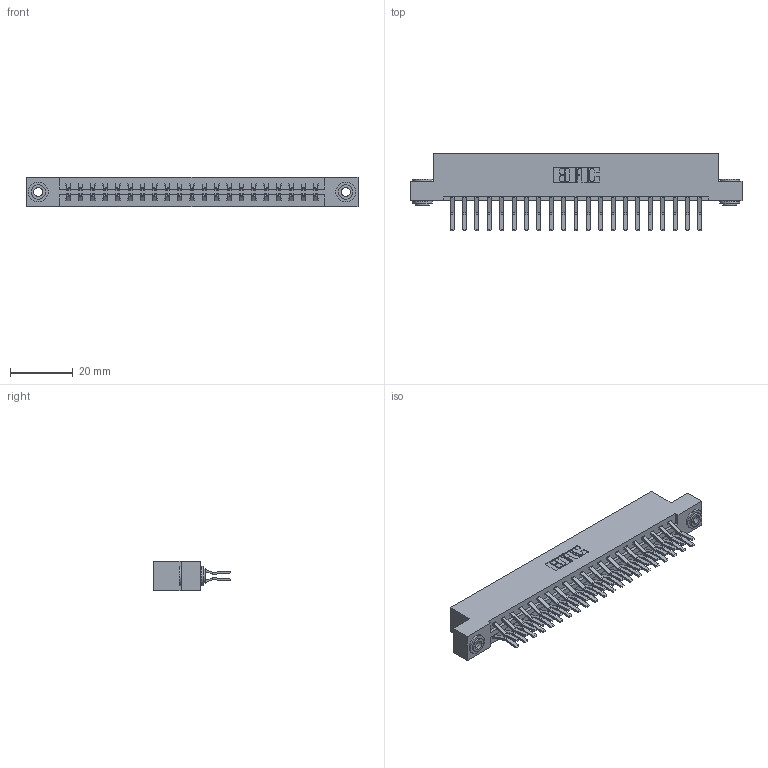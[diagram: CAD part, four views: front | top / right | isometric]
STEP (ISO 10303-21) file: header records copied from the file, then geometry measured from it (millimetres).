
FILE_DESCRIPTION (( 'STEP AP203' ), '1' );
FILE_NAME ('387-042-560-203.STEP', '2019-10-18T04:57:47', ( '' ), ( '' ), 'SwSTEP 2.0', 'SolidWorks 2016', '' );
FILE_SCHEMA (( 'CONFIG_CONTROL_DESIGN' ));
Length unit declared in the file: inch
Products named in the file (4): 337 Part_Flush Mounting Lugs - 0.156 Dia-TH; 387-042-560-203; 345-292-001_560 Tail; 345-250-002_345-250-002-102
Assembly tree (45 placements, depth 2):
  387-042-560-203
    337 Part_Flush Mounting Lugs - 0.156 Dia-TH
    345-292-001_560 Tail  x42
    345-250-002_345-250-002-102  x2
Bounding box: 106.22 x 24.78 x 9.4 mm (x, y, z)
Volume: 11209.8 mm3; surface area: 13489.8 mm2
Topology: 45 solids, 45 shells, 2504 faces, 7401 edges, 4874 vertices
Faces by surface type: plane 1676, cylinder 820, cone 8
Entity records: 19736 total; most frequent: CARTESIAN_POINT 3317, ORIENTED_EDGE 3246, DIRECTION 2897, EDGE_CURVE 1623, LINE 1467, VECTOR 1467, VERTEX_POINT 1078, AXIS2_PLACEMENT_3D 715
